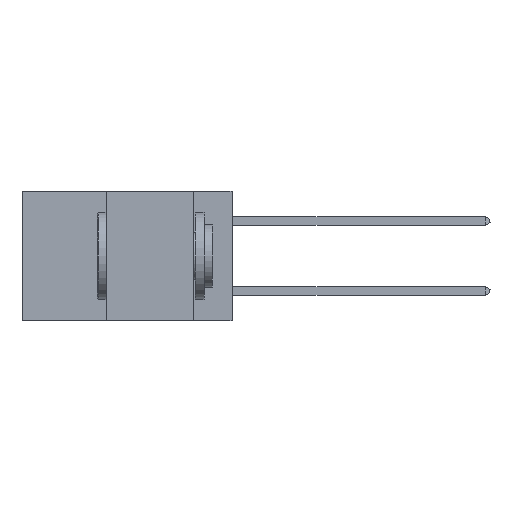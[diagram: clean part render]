
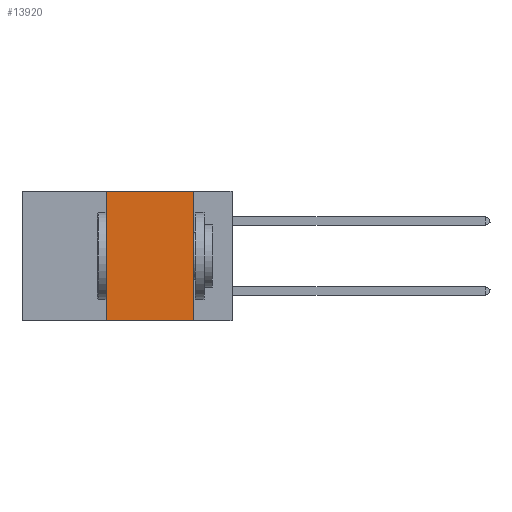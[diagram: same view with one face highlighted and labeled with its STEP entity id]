
A CAD part, left-side view. The second image highlights one B-rep face of the part: STEP entity #13920.
In plain terms, the highlighted planar face has unit normal (-1, 0, 0).
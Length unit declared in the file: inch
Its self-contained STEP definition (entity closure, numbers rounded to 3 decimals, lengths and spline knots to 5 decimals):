
#1502 = LINE ( 'NONE', #5748, #34660 ) ;
#1682 = CARTESIAN_POINT ( 'NONE',  ( 0., 0.6, -0.37 ) ) ;
#3670 = VERTEX_POINT ( 'NONE', #19004 ) ;
#3711 = ORIENTED_EDGE ( 'NONE', *, *, #7338, .F. ) ;
#5748 = CARTESIAN_POINT ( 'NONE',  ( 0., 0.11, 0. ) ) ;
#6284 = VERTEX_POINT ( 'NONE', #33594 ) ;
#7338 = EDGE_CURVE ( 'NONE', #6284, #32142, #1502, .T. ) ;
#8077 = CARTESIAN_POINT ( 'NONE',  ( 0., 0.6, 0. ) ) ;
#8742 = FACE_OUTER_BOUND ( 'NONE', #33403, .T. ) ;
#10167 = LINE ( 'NONE', #28106, #23739 ) ;
#11257 = CARTESIAN_POINT ( 'NONE',  ( 0., 0.36, -0.37 ) ) ;
#13920 = ADVANCED_FACE ( 'NONE', ( #8742 ), #18363, .F. ) ;
#14394 = AXIS2_PLACEMENT_3D ( 'NONE', #41047, #28289, #24774 ) ;
#18125 = LINE ( 'NONE', #1682, #25604 ) ;
#18363 = PLANE ( 'NONE',  #14394 ) ;
#19004 = CARTESIAN_POINT ( 'NONE',  ( 0., 0.36, 0. ) ) ;
#21744 = ORIENTED_EDGE ( 'NONE', *, *, #29271, .F. ) ;
#23739 = VECTOR ( 'NONE', #34413, 39.37008 ) ;
#24774 = DIRECTION ( 'NONE',  ( 0., 0., -1. ) ) ;
#25604 = VECTOR ( 'NONE', #27286, 39.37008 ) ;
#26391 = ORIENTED_EDGE ( 'NONE', *, *, #32975, .T. ) ;
#26516 = LINE ( 'NONE', #8077, #41060 ) ;
#27286 = DIRECTION ( 'NONE',  ( 0., -1., 0. ) ) ;
#28106 = CARTESIAN_POINT ( 'NONE',  ( 0., 0.36, 0. ) ) ;
#28289 = DIRECTION ( 'NONE',  ( 1., 0., 0. ) ) ;
#29271 = EDGE_CURVE ( 'NONE', #35616, #3670, #10167, .T. ) ;
#30535 = DIRECTION ( 'NONE',  ( 0., -1., 0. ) ) ;
#31552 = EDGE_CURVE ( 'NONE', #3670, #6284, #26516, .T. ) ;
#32142 = VERTEX_POINT ( 'NONE', #37371 ) ;
#32975 = EDGE_CURVE ( 'NONE', #35616, #32142, #18125, .T. ) ;
#33403 = EDGE_LOOP ( 'NONE', ( #3711, #38500, #21744, #26391 ) ) ;
#33594 = CARTESIAN_POINT ( 'NONE',  ( 0., 0.11, 0. ) ) ;
#34413 = DIRECTION ( 'NONE',  ( 0., 0., 1. ) ) ;
#34660 = VECTOR ( 'NONE', #40578, 39.37008 ) ;
#35616 = VERTEX_POINT ( 'NONE', #11257 ) ;
#37371 = CARTESIAN_POINT ( 'NONE',  ( 0., 0.11, -0.37 ) ) ;
#38500 = ORIENTED_EDGE ( 'NONE', *, *, #31552, .F. ) ;
#40578 = DIRECTION ( 'NONE',  ( 0., 0., -1. ) ) ;
#41047 = CARTESIAN_POINT ( 'NONE',  ( 0., 0.6, 0. ) ) ;
#41060 = VECTOR ( 'NONE', #30535, 39.37008 ) ;
